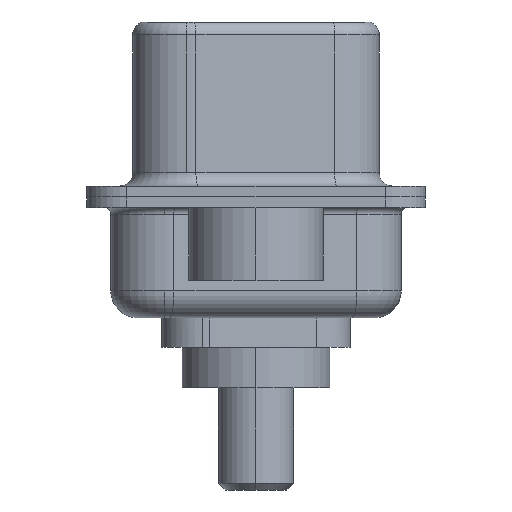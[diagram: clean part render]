
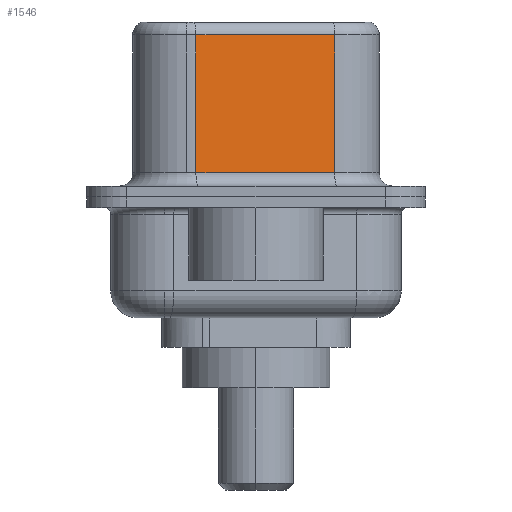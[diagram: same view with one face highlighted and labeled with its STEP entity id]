
A CAD part, left-side view. The second image highlights one B-rep face of the part: STEP entity #1546.
In plain terms, the highlighted planar face has unit normal (-0.985, -0.174, 0).
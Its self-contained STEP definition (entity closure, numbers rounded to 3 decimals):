
#371 = CARTESIAN_POINT ( 'NONE',  ( 4.58, -2.927, 0.9 ) ) ;
#510 = EDGE_LOOP ( 'NONE', ( #2759, #5468, #12512, #7043 ) ) ;
#1546 = ADVANCED_FACE ( 'NONE', ( #3582 ), #4338, .F. ) ;
#1632 = VERTEX_POINT ( 'NONE', #11893 ) ;
#2293 = EDGE_CURVE ( 'NONE', #11118, #10257, #9992, .T. ) ;
#2759 = ORIENTED_EDGE ( 'NONE', *, *, #2293, .F. ) ;
#2812 = LINE ( 'NONE', #5720, #8359 ) ;
#3163 = CARTESIAN_POINT ( 'NONE',  ( 4.58, -2.927, 6.02 ) ) ;
#3288 = EDGE_CURVE ( 'NONE', #1632, #10257, #8683, .T. ) ;
#3582 = FACE_OUTER_BOUND ( 'NONE', #510, .T. ) ;
#4338 = PLANE ( 'NONE',  #10030 ) ;
#4370 = VECTOR ( 'NONE', #7176, 1000. ) ;
#4876 = CARTESIAN_POINT ( 'NONE',  ( 4.58, -2.927, 6.52 ) ) ;
#5033 = DIRECTION ( 'NONE',  ( -0.174, 0.985, 0. ) ) ;
#5172 = VECTOR ( 'NONE', #5033, 1000. ) ;
#5468 = ORIENTED_EDGE ( 'NONE', *, *, #7110, .T. ) ;
#5521 = VECTOR ( 'NONE', #14162, 1000. ) ;
#5549 = DIRECTION ( 'NONE',  ( 0., 0., -1. ) ) ;
#5720 = CARTESIAN_POINT ( 'NONE',  ( 3.67, 2.233, 6.52 ) ) ;
#7043 = ORIENTED_EDGE ( 'NONE', *, *, #3288, .T. ) ;
#7110 = EDGE_CURVE ( 'NONE', #11118, #13928, #8276, .T. ) ;
#7176 = DIRECTION ( 'NONE',  ( 0., 0., -1. ) ) ;
#8276 = LINE ( 'NONE', #3163, #5172 ) ;
#8318 = DIRECTION ( 'NONE',  ( -0.174, 0.985, 0. ) ) ;
#8359 = VECTOR ( 'NONE', #5549, 1000. ) ;
#8683 = LINE ( 'NONE', #371, #5521 ) ;
#8764 = EDGE_CURVE ( 'NONE', #13928, #1632, #2812, .T. ) ;
#8841 = CARTESIAN_POINT ( 'NONE',  ( 4.58, -2.927, 6.52 ) ) ;
#9380 = CARTESIAN_POINT ( 'NONE',  ( 4.58, -2.927, 6.02 ) ) ;
#9985 = CARTESIAN_POINT ( 'NONE',  ( 3.67, 2.233, 6.02 ) ) ;
#9992 = LINE ( 'NONE', #8841, #4370 ) ;
#10030 = AXIS2_PLACEMENT_3D ( 'NONE', #4876, #12253, #8318 ) ;
#10257 = VERTEX_POINT ( 'NONE', #10991 ) ;
#10991 = CARTESIAN_POINT ( 'NONE',  ( 4.58, -2.927, 0.9 ) ) ;
#11118 = VERTEX_POINT ( 'NONE', #9380 ) ;
#11893 = CARTESIAN_POINT ( 'NONE',  ( 3.67, 2.233, 0.9 ) ) ;
#12253 = DIRECTION ( 'NONE',  ( 0.985, 0.174, 0. ) ) ;
#12512 = ORIENTED_EDGE ( 'NONE', *, *, #8764, .T. ) ;
#13928 = VERTEX_POINT ( 'NONE', #9985 ) ;
#14162 = DIRECTION ( 'NONE',  ( 0.174, -0.985, 0. ) ) ;
